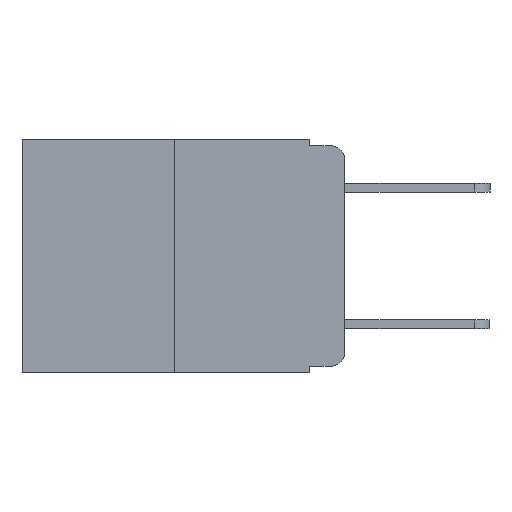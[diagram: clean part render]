
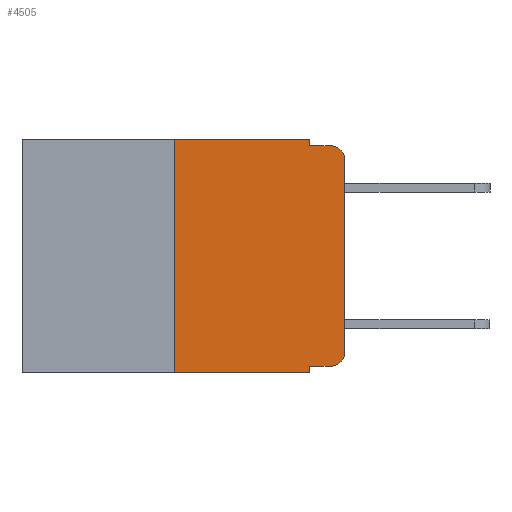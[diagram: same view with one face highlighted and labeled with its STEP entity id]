
A CAD part, left-side view. The second image highlights one B-rep face of the part: STEP entity #4505.
In plain terms, the highlighted planar face has unit normal (-1, 0, 0).
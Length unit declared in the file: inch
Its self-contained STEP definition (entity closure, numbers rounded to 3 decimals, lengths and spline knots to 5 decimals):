
#891 = ORIENTED_EDGE ( 'NONE', *, *, #19517, .F. ) ;
#1108 = CARTESIAN_POINT ( 'NONE',  ( 0., 0.25, 0. ) ) ;
#1141 = AXIS2_PLACEMENT_3D ( 'NONE', #8431, #21666, #10324 ) ;
#1215 = DIRECTION ( 'NONE',  ( -1., 0., 0. ) ) ;
#1597 = ORIENTED_EDGE ( 'NONE', *, *, #11206, .F. ) ;
#1849 = CARTESIAN_POINT ( 'NONE',  ( 0., 0.473, 0. ) ) ;
#1926 = VERTEX_POINT ( 'NONE', #12530 ) ;
#2971 = CARTESIAN_POINT ( 'NONE',  ( 0., 0.25, 0. ) ) ;
#3739 = CARTESIAN_POINT ( 'NONE',  ( 0., 0., 0. ) ) ;
#4505 = ADVANCED_FACE ( 'NONE', ( #17308 ), #15866, .F. ) ;
#5659 = LINE ( 'NONE', #10533, #19684 ) ;
#5741 = VECTOR ( 'NONE', #14584, 39.37008 ) ;
#6068 = EDGE_CURVE ( 'NONE', #25055, #16664, #20583, .T. ) ;
#6387 = VECTOR ( 'NONE', #20863, 39.37008 ) ;
#6390 = LINE ( 'NONE', #3739, #15232 ) ;
#6547 = VERTEX_POINT ( 'NONE', #16285 ) ;
#7018 = DIRECTION ( 'NONE',  ( -1., 0., 0. ) ) ;
#7399 = EDGE_CURVE ( 'NONE', #11554, #25055, #16568, .T. ) ;
#7476 = VECTOR ( 'NONE', #11044, 39.37008 ) ;
#7629 = CARTESIAN_POINT ( 'NONE',  ( 0., 0.051, 0. ) ) ;
#8431 = CARTESIAN_POINT ( 'NONE',  ( 0., 0.473, 0. ) ) ;
#9020 = CARTESIAN_POINT ( 'NONE',  ( 0., 0.02, -0.01 ) ) ;
#9043 = CARTESIAN_POINT ( 'NONE',  ( 0., 0.051, 0. ) ) ;
#9240 = CARTESIAN_POINT ( 'NONE',  ( 0., 0.02, -0.333 ) ) ;
#9355 = VERTEX_POINT ( 'NONE', #14111 ) ;
#9862 = VERTEX_POINT ( 'NONE', #9020 ) ;
#10029 = ORIENTED_EDGE ( 'NONE', *, *, #12470, .F. ) ;
#10324 = DIRECTION ( 'NONE',  ( 0., 0., -1. ) ) ;
#10356 = ORIENTED_EDGE ( 'NONE', *, *, #7399, .T. ) ;
#10432 = CIRCLE ( 'NONE', #18848, 0.02 ) ;
#10512 = CARTESIAN_POINT ( 'NONE',  ( 0., 0.051, -0.333 ) ) ;
#10533 = CARTESIAN_POINT ( 'NONE',  ( 0., 0.473, -0.343 ) ) ;
#10864 = LINE ( 'NONE', #9043, #5741 ) ;
#10892 = ORIENTED_EDGE ( 'NONE', *, *, #14949, .F. ) ;
#10901 = CARTESIAN_POINT ( 'NONE',  ( 0., 0.051, -0.01 ) ) ;
#11044 = DIRECTION ( 'NONE',  ( 0., 0., 1. ) ) ;
#11165 = AXIS2_PLACEMENT_3D ( 'NONE', #18315, #7018, #20283 ) ;
#11206 = EDGE_CURVE ( 'NONE', #11554, #20151, #14650, .T. ) ;
#11531 = ORIENTED_EDGE ( 'NONE', *, *, #6068, .T. ) ;
#11554 = VERTEX_POINT ( 'NONE', #10512 ) ;
#11757 = CARTESIAN_POINT ( 'NONE',  ( 0., 0.051, -0.343 ) ) ;
#12417 = DIRECTION ( 'NONE',  ( 0., -1., 0. ) ) ;
#12470 = EDGE_CURVE ( 'NONE', #1926, #18699, #12498, .T. ) ;
#12498 = LINE ( 'NONE', #1108, #7476 ) ;
#12530 = CARTESIAN_POINT ( 'NONE',  ( 0., 0.25, -0.343 ) ) ;
#13037 = CARTESIAN_POINT ( 'NONE',  ( 0., 0.02, -0.03 ) ) ;
#14111 = CARTESIAN_POINT ( 'NONE',  ( 0., 0.051, -0.01 ) ) ;
#14404 = EDGE_LOOP ( 'NONE', ( #21490, #23298, #24171, #10892, #891, #10029, #19204, #1597, #10356, #11531 ) ) ;
#14584 = DIRECTION ( 'NONE',  ( 0., 0., -1. ) ) ;
#14650 = LINE ( 'NONE', #7629, #6387 ) ;
#14889 = DIRECTION ( 'NONE',  ( 0., 0., -1. ) ) ;
#14949 = EDGE_CURVE ( 'NONE', #6547, #9355, #10864, .T. ) ;
#15164 = VECTOR ( 'NONE', #22238, 39.37008 ) ;
#15232 = VECTOR ( 'NONE', #19147, 39.37008 ) ;
#15388 = CARTESIAN_POINT ( 'NONE',  ( 0., 0.051, -0.333 ) ) ;
#15477 = DIRECTION ( 'NONE',  ( 0., -1., 0. ) ) ;
#15866 = PLANE ( 'NONE',  #1141 ) ;
#16205 = EDGE_CURVE ( 'NONE', #9355, #9862, #20289, .T. ) ;
#16285 = CARTESIAN_POINT ( 'NONE',  ( 0., 0.051, 0. ) ) ;
#16568 = LINE ( 'NONE', #15388, #21088 ) ;
#16664 = VERTEX_POINT ( 'NONE', #24553 ) ;
#17308 = FACE_OUTER_BOUND ( 'NONE', #14404, .T. ) ;
#17326 = DIRECTION ( 'NONE',  ( 0., -1., 0. ) ) ;
#18315 = CARTESIAN_POINT ( 'NONE',  ( 0., 0.02, -0.313 ) ) ;
#18329 = VECTOR ( 'NONE', #17326, 39.37008 ) ;
#18699 = VERTEX_POINT ( 'NONE', #2971 ) ;
#18808 = EDGE_CURVE ( 'NONE', #22876, #9862, #10432, .T. ) ;
#18848 = AXIS2_PLACEMENT_3D ( 'NONE', #13037, #1215, #14889 ) ;
#18960 = LINE ( 'NONE', #1849, #18329 ) ;
#19147 = DIRECTION ( 'NONE',  ( 0., 0., 1. ) ) ;
#19204 = ORIENTED_EDGE ( 'NONE', *, *, #23723, .T. ) ;
#19517 = EDGE_CURVE ( 'NONE', #18699, #6547, #18960, .T. ) ;
#19684 = VECTOR ( 'NONE', #12417, 39.37008 ) ;
#20151 = VERTEX_POINT ( 'NONE', #11757 ) ;
#20283 = DIRECTION ( 'NONE',  ( 0., 0., -1. ) ) ;
#20289 = LINE ( 'NONE', #10901, #15164 ) ;
#20583 = CIRCLE ( 'NONE', #11165, 0.02 ) ;
#20863 = DIRECTION ( 'NONE',  ( 0., 0., -1. ) ) ;
#21058 = CARTESIAN_POINT ( 'NONE',  ( 0., 0., -0.03 ) ) ;
#21088 = VECTOR ( 'NONE', #15477, 39.37008 ) ;
#21355 = EDGE_CURVE ( 'NONE', #16664, #22876, #6390, .T. ) ;
#21490 = ORIENTED_EDGE ( 'NONE', *, *, #21355, .T. ) ;
#21666 = DIRECTION ( 'NONE',  ( 1., 0., 0. ) ) ;
#22238 = DIRECTION ( 'NONE',  ( 0., -1., 0. ) ) ;
#22876 = VERTEX_POINT ( 'NONE', #21058 ) ;
#23298 = ORIENTED_EDGE ( 'NONE', *, *, #18808, .T. ) ;
#23723 = EDGE_CURVE ( 'NONE', #1926, #20151, #5659, .T. ) ;
#24171 = ORIENTED_EDGE ( 'NONE', *, *, #16205, .F. ) ;
#24553 = CARTESIAN_POINT ( 'NONE',  ( 0., 0., -0.313 ) ) ;
#25055 = VERTEX_POINT ( 'NONE', #9240 ) ;
